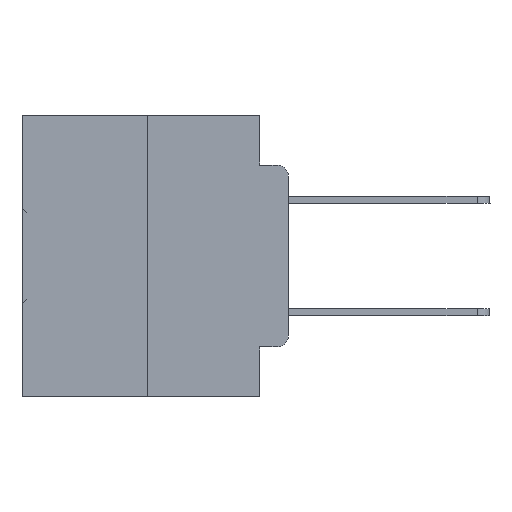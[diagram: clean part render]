
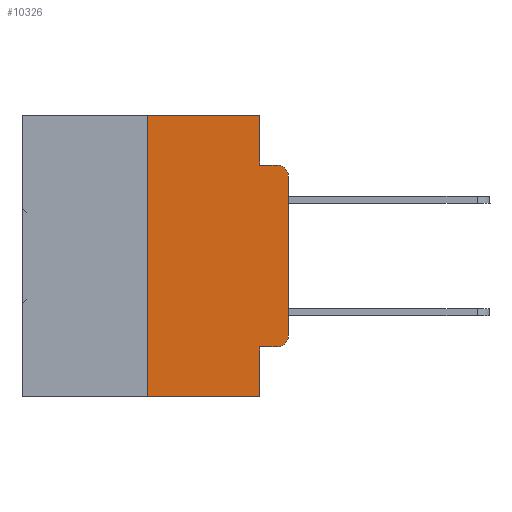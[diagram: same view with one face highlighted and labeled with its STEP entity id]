
A CAD part, left-side view. The second image highlights one B-rep face of the part: STEP entity #10326.
In plain terms, the highlighted planar face has unit normal (-1, 0, 0).
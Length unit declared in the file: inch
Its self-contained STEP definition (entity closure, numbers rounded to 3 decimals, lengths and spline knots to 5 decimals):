
#425 = VERTEX_POINT ( 'NONE', #23285 ) ;
#643 = VECTOR ( 'NONE', #7978, 39.37008 ) ;
#646 = DIRECTION ( 'NONE',  ( 0., 0., -1. ) ) ;
#869 = DIRECTION ( 'NONE',  ( 0., 0., -1. ) ) ;
#952 = LINE ( 'NONE', #28209, #14415 ) ;
#1802 = ORIENTED_EDGE ( 'NONE', *, *, #25954, .T. ) ;
#4108 = DIRECTION ( 'NONE',  ( 0., 0., 1. ) ) ;
#4381 = EDGE_LOOP ( 'NONE', ( #20135, #22021, #33384, #27347, #34404, #13226, #1802, #24221, #12859, #32384 ) ) ;
#4390 = EDGE_CURVE ( 'NONE', #10950, #30279, #33301, .T. ) ;
#6546 = EDGE_CURVE ( 'NONE', #25506, #8526, #14325, .T. ) ;
#7766 = VERTEX_POINT ( 'NONE', #18262 ) ;
#7978 = DIRECTION ( 'NONE',  ( 0., -1., 0. ) ) ;
#8421 = VERTEX_POINT ( 'NONE', #19293 ) ;
#8526 = VERTEX_POINT ( 'NONE', #19640 ) ;
#8866 = CARTESIAN_POINT ( 'NONE',  ( 0., 0.051, -0.0885 ) ) ;
#9027 = CARTESIAN_POINT ( 'NONE',  ( 0., 0., -0.1085 ) ) ;
#10326 = ADVANCED_FACE ( 'NONE', ( #14856 ), #21135, .F. ) ;
#10441 = VECTOR ( 'NONE', #25111, 39.37008 ) ;
#10668 = CARTESIAN_POINT ( 'NONE',  ( 0., 0., 0. ) ) ;
#10950 = VERTEX_POINT ( 'NONE', #16174 ) ;
#11379 = CARTESIAN_POINT ( 'NONE',  ( 0., 0.25, -0.5 ) ) ;
#12859 = ORIENTED_EDGE ( 'NONE', *, *, #21043, .T. ) ;
#13226 = ORIENTED_EDGE ( 'NONE', *, *, #15086, .F. ) ;
#13438 = CARTESIAN_POINT ( 'NONE',  ( 0., 0.473, 0. ) ) ;
#13853 = LINE ( 'NONE', #24589, #19092 ) ;
#14325 = LINE ( 'NONE', #8866, #18160 ) ;
#14415 = VECTOR ( 'NONE', #4108, 39.37008 ) ;
#14423 = VERTEX_POINT ( 'NONE', #11379 ) ;
#14856 = FACE_OUTER_BOUND ( 'NONE', #4381, .T. ) ;
#15055 = AXIS2_PLACEMENT_3D ( 'NONE', #27356, #16289, #646 ) ;
#15086 = EDGE_CURVE ( 'NONE', #14423, #34349, #952, .T. ) ;
#15579 = VECTOR ( 'NONE', #29181, 39.37008 ) ;
#15708 = CARTESIAN_POINT ( 'NONE',  ( 0., 0.25, 0. ) ) ;
#15762 = EDGE_CURVE ( 'NONE', #7766, #25506, #29528, .T. ) ;
#15847 = VECTOR ( 'NONE', #32125, 39.37008 ) ;
#16174 = CARTESIAN_POINT ( 'NONE',  ( 0., 0.02, -0.4115 ) ) ;
#16289 = DIRECTION ( 'NONE',  ( -1., 0., 0. ) ) ;
#16711 = CARTESIAN_POINT ( 'NONE',  ( 0., 0.051, -0.4115 ) ) ;
#17721 = CARTESIAN_POINT ( 'NONE',  ( 0., 0.473, -0.5 ) ) ;
#17869 = CIRCLE ( 'NONE', #15055, 0.02 ) ;
#18160 = VECTOR ( 'NONE', #19946, 39.37008 ) ;
#18262 = CARTESIAN_POINT ( 'NONE',  ( 0., 0.051, 0. ) ) ;
#18348 = CARTESIAN_POINT ( 'NONE',  ( 0., 0.473, 0. ) ) ;
#18940 = VERTEX_POINT ( 'NONE', #9027 ) ;
#18995 = CARTESIAN_POINT ( 'NONE',  ( 0., 0.051, -0.0885 ) ) ;
#19092 = VECTOR ( 'NONE', #32660, 39.37008 ) ;
#19150 = VECTOR ( 'NONE', #30067, 39.37008 ) ;
#19293 = CARTESIAN_POINT ( 'NONE',  ( 0., 0.051, -0.4115 ) ) ;
#19346 = LINE ( 'NONE', #16711, #19150 ) ;
#19640 = CARTESIAN_POINT ( 'NONE',  ( 0., 0.02, -0.0885 ) ) ;
#19946 = DIRECTION ( 'NONE',  ( 0., -1., 0. ) ) ;
#20135 = ORIENTED_EDGE ( 'NONE', *, *, #33752, .T. ) ;
#21043 = EDGE_CURVE ( 'NONE', #8421, #10950, #19346, .T. ) ;
#21135 = PLANE ( 'NONE',  #28448 ) ;
#21491 = EDGE_CURVE ( 'NONE', #8421, #425, #13853, .T. ) ;
#22021 = ORIENTED_EDGE ( 'NONE', *, *, #27592, .T. ) ;
#22655 = DIRECTION ( 'NONE',  ( -1., 0., 0. ) ) ;
#23285 = CARTESIAN_POINT ( 'NONE',  ( 0., 0.051, -0.5 ) ) ;
#23628 = DIRECTION ( 'NONE',  ( 1., 0., 0. ) ) ;
#24030 = LINE ( 'NONE', #10668, #15847 ) ;
#24221 = ORIENTED_EDGE ( 'NONE', *, *, #21491, .F. ) ;
#24589 = CARTESIAN_POINT ( 'NONE',  ( 0., 0.051, 0. ) ) ;
#25111 = DIRECTION ( 'NONE',  ( 0., -1., 0. ) ) ;
#25313 = CARTESIAN_POINT ( 'NONE',  ( 0., 0.02, -0.3915 ) ) ;
#25506 = VERTEX_POINT ( 'NONE', #18995 ) ;
#25954 = EDGE_CURVE ( 'NONE', #14423, #425, #30562, .T. ) ;
#26114 = CARTESIAN_POINT ( 'NONE',  ( 0., 0., -0.3915 ) ) ;
#27347 = ORIENTED_EDGE ( 'NONE', *, *, #15762, .F. ) ;
#27356 = CARTESIAN_POINT ( 'NONE',  ( 0., 0.02, -0.1085 ) ) ;
#27592 = EDGE_CURVE ( 'NONE', #18940, #8526, #17869, .T. ) ;
#28209 = CARTESIAN_POINT ( 'NONE',  ( 0., 0.25, 0. ) ) ;
#28448 = AXIS2_PLACEMENT_3D ( 'NONE', #18348, #23628, #34487 ) ;
#29006 = CARTESIAN_POINT ( 'NONE',  ( 0., 0.051, 0. ) ) ;
#29181 = DIRECTION ( 'NONE',  ( 0., 0., -1. ) ) ;
#29528 = LINE ( 'NONE', #29006, #15579 ) ;
#30067 = DIRECTION ( 'NONE',  ( 0., -1., 0. ) ) ;
#30279 = VERTEX_POINT ( 'NONE', #26114 ) ;
#30562 = LINE ( 'NONE', #17721, #10441 ) ;
#32076 = LINE ( 'NONE', #13438, #643 ) ;
#32125 = DIRECTION ( 'NONE',  ( 0., 0., 1. ) ) ;
#32384 = ORIENTED_EDGE ( 'NONE', *, *, #4390, .T. ) ;
#32660 = DIRECTION ( 'NONE',  ( 0., 0., -1. ) ) ;
#32952 = EDGE_CURVE ( 'NONE', #34349, #7766, #32076, .T. ) ;
#33301 = CIRCLE ( 'NONE', #34384, 0.02 ) ;
#33384 = ORIENTED_EDGE ( 'NONE', *, *, #6546, .F. ) ;
#33752 = EDGE_CURVE ( 'NONE', #30279, #18940, #24030, .T. ) ;
#34349 = VERTEX_POINT ( 'NONE', #15708 ) ;
#34384 = AXIS2_PLACEMENT_3D ( 'NONE', #25313, #22655, #869 ) ;
#34404 = ORIENTED_EDGE ( 'NONE', *, *, #32952, .F. ) ;
#34487 = DIRECTION ( 'NONE',  ( 0., 0., -1. ) ) ;
